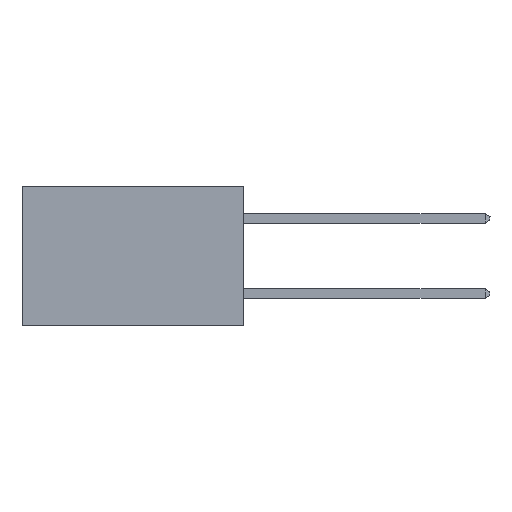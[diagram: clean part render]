
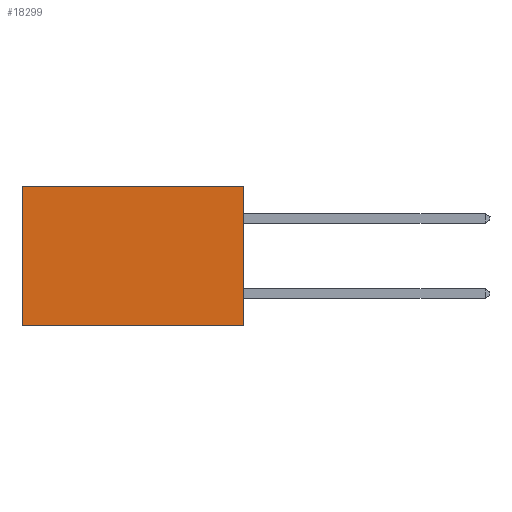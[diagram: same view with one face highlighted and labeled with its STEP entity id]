
A CAD part, left-side view. The second image highlights one B-rep face of the part: STEP entity #18299.
In plain terms, the highlighted planar face has unit normal (-1, 0, 0).
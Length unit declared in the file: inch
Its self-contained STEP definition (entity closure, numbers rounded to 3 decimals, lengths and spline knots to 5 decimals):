
#2030 = CARTESIAN_POINT ( 'NONE',  ( 0.277, 0., 0. ) ) ;
#2281 = DIRECTION ( 'NONE',  ( 0., 0., -1. ) ) ;
#2856 = EDGE_CURVE ( 'NONE', #28139, #20892, #20710, .T. ) ;
#2980 = VECTOR ( 'NONE', #8821, 39.37008 ) ;
#4068 = VERTEX_POINT ( 'NONE', #6932 ) ;
#4269 = VECTOR ( 'NONE', #26624, 39.37008 ) ;
#4710 = VECTOR ( 'NONE', #2281, 39.37008 ) ;
#6860 = EDGE_LOOP ( 'NONE', ( #28106, #27507, #27647, #27177 ) ) ;
#6895 = PLANE ( 'NONE',  #11797 ) ;
#6932 = CARTESIAN_POINT ( 'NONE',  ( 0.277, 0., 0. ) ) ;
#8821 = DIRECTION ( 'NONE',  ( 0., 1., 0. ) ) ;
#9134 = DIRECTION ( 'NONE',  ( 1., 0., 0. ) ) ;
#11528 = CARTESIAN_POINT ( 'NONE',  ( 0.277, 0.59, -0.37 ) ) ;
#11797 = AXIS2_PLACEMENT_3D ( 'NONE', #22018, #9134, #24154 ) ;
#11843 = DIRECTION ( 'NONE',  ( 0., 0., -1. ) ) ;
#14752 = EDGE_CURVE ( 'NONE', #23576, #20892, #21613, .T. ) ;
#15081 = FACE_OUTER_BOUND ( 'NONE', #6860, .T. ) ;
#15841 = CARTESIAN_POINT ( 'NONE',  ( 0.277, 0.59, -0.37 ) ) ;
#16050 = CARTESIAN_POINT ( 'NONE',  ( 0.277, 0., -0.37 ) ) ;
#16378 = LINE ( 'NONE', #19838, #4710 ) ;
#18299 = ADVANCED_FACE ( 'NONE', ( #15081 ), #6895, .F. ) ;
#19838 = CARTESIAN_POINT ( 'NONE',  ( 0.277, 0., -0.37 ) ) ;
#20458 = LINE ( 'NONE', #2030, #2980 ) ;
#20710 = LINE ( 'NONE', #15841, #26383 ) ;
#20892 = VERTEX_POINT ( 'NONE', #11528 ) ;
#21578 = CARTESIAN_POINT ( 'NONE',  ( 0.277, 0.59, 0. ) ) ;
#21613 = LINE ( 'NONE', #24440, #4269 ) ;
#22018 = CARTESIAN_POINT ( 'NONE',  ( 0.277, 0., -0.37 ) ) ;
#23314 = EDGE_CURVE ( 'NONE', #4068, #28139, #20458, .T. ) ;
#23576 = VERTEX_POINT ( 'NONE', #16050 ) ;
#24154 = DIRECTION ( 'NONE',  ( 0., 0., -1. ) ) ;
#24382 = EDGE_CURVE ( 'NONE', #4068, #23576, #16378, .T. ) ;
#24440 = CARTESIAN_POINT ( 'NONE',  ( 0.277, 0., -0.37 ) ) ;
#26383 = VECTOR ( 'NONE', #11843, 39.37008 ) ;
#26624 = DIRECTION ( 'NONE',  ( 0., 1., 0. ) ) ;
#27177 = ORIENTED_EDGE ( 'NONE', *, *, #23314, .T. ) ;
#27507 = ORIENTED_EDGE ( 'NONE', *, *, #14752, .F. ) ;
#27647 = ORIENTED_EDGE ( 'NONE', *, *, #24382, .F. ) ;
#28106 = ORIENTED_EDGE ( 'NONE', *, *, #2856, .T. ) ;
#28139 = VERTEX_POINT ( 'NONE', #21578 ) ;
